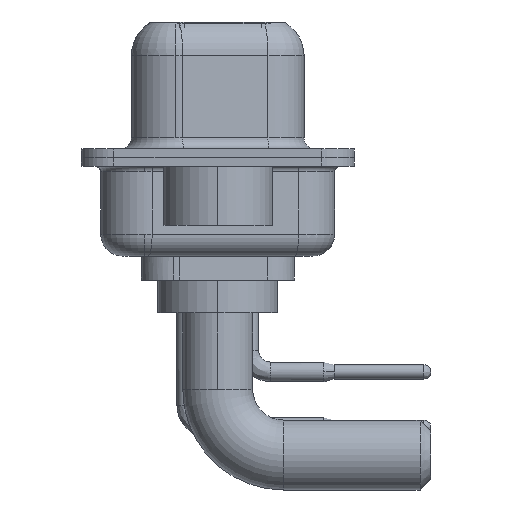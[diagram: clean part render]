
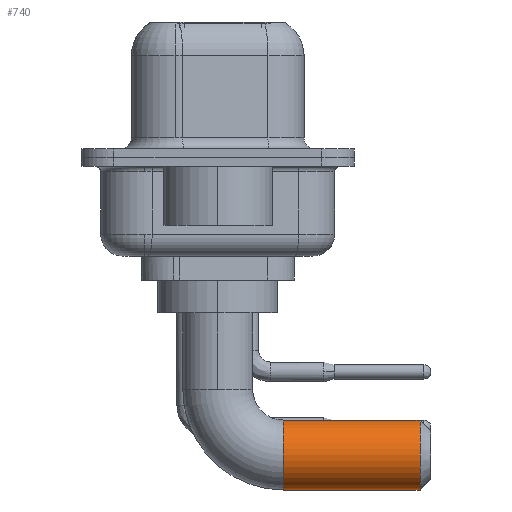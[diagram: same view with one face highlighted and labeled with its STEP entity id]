
A CAD part, left-side view. The second image highlights one B-rep face of the part: STEP entity #740.
In plain terms, the highlighted cylindrical face has radius 1.6 mm (diameter 3.2 mm), a partial arc.
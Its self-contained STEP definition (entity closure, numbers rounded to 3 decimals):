
#740 = ADVANCED_FACE ( 'NONE', ( #2737 ), #18474, .T. ) ;
#819 = EDGE_CURVE ( 'NONE', #8977, #7318, #12123, .T. ) ;
#835 = CARTESIAN_POINT ( 'NONE',  ( 0., -3., -6.5 ) ) ;
#1470 = VECTOR ( 'NONE', #9219, 1000. ) ;
#2607 = ORIENTED_EDGE ( 'NONE', *, *, #819, .T. ) ;
#2634 = VERTEX_POINT ( 'NONE', #4383 ) ;
#2737 = FACE_OUTER_BOUND ( 'NONE', #3600, .T. ) ;
#2978 = CARTESIAN_POINT ( 'NONE',  ( 0., -3., -8.1 ) ) ;
#3317 = AXIS2_PLACEMENT_3D ( 'NONE', #10813, #7446, #12348 ) ;
#3600 = EDGE_LOOP ( 'NONE', ( #18836, #2607, #18196, #9278 ) ) ;
#3949 = VERTEX_POINT ( 'NONE', #15550 ) ;
#4269 = DIRECTION ( 'NONE',  ( 0., -1., 0. ) ) ;
#4383 = CARTESIAN_POINT ( 'NONE',  ( 0., -9.25, -8.1 ) ) ;
#5279 = EDGE_CURVE ( 'NONE', #7318, #2634, #10753, .T. ) ;
#5443 = CARTESIAN_POINT ( 'NONE',  ( 0., -9.25, -6.5 ) ) ;
#6259 = LINE ( 'NONE', #12503, #10868 ) ;
#6832 = EDGE_CURVE ( 'NONE', #2634, #3949, #16856, .T. ) ;
#7318 = VERTEX_POINT ( 'NONE', #13083 ) ;
#7446 = DIRECTION ( 'NONE',  ( 0., -1., 0. ) ) ;
#8203 = AXIS2_PLACEMENT_3D ( 'NONE', #835, #4269, #15213 ) ;
#8977 = VERTEX_POINT ( 'NONE', #14238 ) ;
#9219 = DIRECTION ( 'NONE',  ( 0., -1., 0. ) ) ;
#9278 = ORIENTED_EDGE ( 'NONE', *, *, #6832, .T. ) ;
#9677 = AXIS2_PLACEMENT_3D ( 'NONE', #5443, #13016, #9942 ) ;
#9942 = DIRECTION ( 'NONE',  ( 0., 0., -1. ) ) ;
#10753 = LINE ( 'NONE', #2978, #1470 ) ;
#10813 = CARTESIAN_POINT ( 'NONE',  ( 0., -3., -6.5 ) ) ;
#10868 = VECTOR ( 'NONE', #15757, 1000. ) ;
#12123 = CIRCLE ( 'NONE', #3317, 1.6 ) ;
#12348 = DIRECTION ( 'NONE',  ( -1., 0., 0. ) ) ;
#12503 = CARTESIAN_POINT ( 'NONE',  ( 0., -3., -4.9 ) ) ;
#13016 = DIRECTION ( 'NONE',  ( 0., 1., 0. ) ) ;
#13083 = CARTESIAN_POINT ( 'NONE',  ( 0., -3., -8.1 ) ) ;
#14238 = CARTESIAN_POINT ( 'NONE',  ( 0., -3., -4.9 ) ) ;
#15213 = DIRECTION ( 'NONE',  ( 0., 0., -1. ) ) ;
#15550 = CARTESIAN_POINT ( 'NONE',  ( 0., -9.25, -4.9 ) ) ;
#15757 = DIRECTION ( 'NONE',  ( 0., -1., 0. ) ) ;
#16856 = CIRCLE ( 'NONE', #9677, 1.6 ) ;
#18196 = ORIENTED_EDGE ( 'NONE', *, *, #5279, .T. ) ;
#18474 = CYLINDRICAL_SURFACE ( 'NONE', #8203, 1.6 ) ;
#18836 = ORIENTED_EDGE ( 'NONE', *, *, #18940, .F. ) ;
#18940 = EDGE_CURVE ( 'NONE', #8977, #3949, #6259, .T. ) ;
